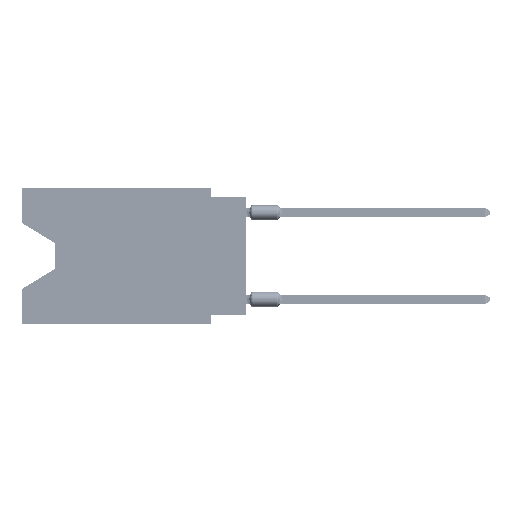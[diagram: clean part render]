
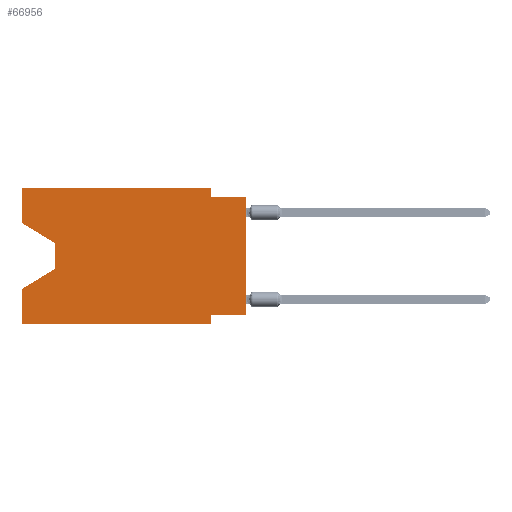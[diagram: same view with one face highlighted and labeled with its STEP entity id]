
A CAD part, left-side view. The second image highlights one B-rep face of the part: STEP entity #66956.
In plain terms, the highlighted planar face has unit normal (-1, 0, 0).
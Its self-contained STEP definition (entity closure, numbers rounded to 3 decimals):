
#85 = ORIENTED_EDGE ( 'NONE', *, *, #61911, .T. ) ;
#291 = CARTESIAN_POINT ( 'NONE',  ( 0., 2.54, 0. ) ) ;
#865 = LINE ( 'NONE', #1725, #47856 ) ;
#953 = ORIENTED_EDGE ( 'NONE', *, *, #16409, .F. ) ;
#1725 = CARTESIAN_POINT ( 'NONE',  ( 0., 2.54, -9.906 ) ) ;
#3393 = ORIENTED_EDGE ( 'NONE', *, *, #36086, .F. ) ;
#3420 = LINE ( 'NONE', #84178, #83410 ) ;
#5322 = CARTESIAN_POINT ( 'NONE',  ( 0., 13.97, -4.013 ) ) ;
#5913 = DIRECTION ( 'NONE',  ( 0., 0., -1. ) ) ;
#6177 = DIRECTION ( 'NONE',  ( 0., 0., -1. ) ) ;
#7702 = CARTESIAN_POINT ( 'NONE',  ( 0., 0., -0.635 ) ) ;
#8508 = DIRECTION ( 'NONE',  ( 0., -0.855, -0.519 ) ) ;
#9386 = CARTESIAN_POINT ( 'NONE',  ( 0., 0., 0. ) ) ;
#10433 = EDGE_CURVE ( 'NONE', #34516, #54500, #32031, .T. ) ;
#11161 = CARTESIAN_POINT ( 'NONE',  ( 0., 2.54, 0. ) ) ;
#11416 = LINE ( 'NONE', #5322, #69441 ) ;
#11665 = VECTOR ( 'NONE', #34186, 1000. ) ;
#12530 = VERTEX_POINT ( 'NONE', #73570 ) ;
#13395 = VECTOR ( 'NONE', #21501, 1000. ) ;
#13916 = DIRECTION ( 'NONE',  ( 0., 0., -1. ) ) ;
#15019 = CARTESIAN_POINT ( 'NONE',  ( 0., 16.383, -2.546 ) ) ;
#16210 = EDGE_CURVE ( 'NONE', #38763, #74793, #22685, .T. ) ;
#16409 = EDGE_CURVE ( 'NONE', #73768, #19472, #865, .T. ) ;
#19472 = VERTEX_POINT ( 'NONE', #46009 ) ;
#21501 = DIRECTION ( 'NONE',  ( 0., 0., 1. ) ) ;
#21680 = VECTOR ( 'NONE', #58626, 1000. ) ;
#22216 = ORIENTED_EDGE ( 'NONE', *, *, #10433, .F. ) ;
#22685 = LINE ( 'NONE', #36582, #36771 ) ;
#24603 = CARTESIAN_POINT ( 'NONE',  ( 0., 0., -0.635 ) ) ;
#25731 = VECTOR ( 'NONE', #8508, 1000. ) ;
#26202 = VERTEX_POINT ( 'NONE', #66694 ) ;
#26262 = EDGE_CURVE ( 'NONE', #26202, #38763, #81428, .T. ) ;
#26643 = CARTESIAN_POINT ( 'NONE',  ( 0., 16.383, -9.906 ) ) ;
#27681 = DIRECTION ( 'NONE',  ( 0., 0., -1. ) ) ;
#28984 = VERTEX_POINT ( 'NONE', #60404 ) ;
#29018 = VECTOR ( 'NONE', #39448, 1000. ) ;
#30464 = ORIENTED_EDGE ( 'NONE', *, *, #26262, .F. ) ;
#31731 = ORIENTED_EDGE ( 'NONE', *, *, #72070, .T. ) ;
#32031 = LINE ( 'NONE', #58087, #45026 ) ;
#32732 = EDGE_LOOP ( 'NONE', ( #79711, #31731, #55553, #22216, #79276, #953, #46967, #85, #33326, #3393, #66245, #30464 ) ) ;
#33326 = ORIENTED_EDGE ( 'NONE', *, *, #43011, .F. ) ;
#33374 = VERTEX_POINT ( 'NONE', #85211 ) ;
#34186 = DIRECTION ( 'NONE',  ( 0., -1., 0. ) ) ;
#34516 = VERTEX_POINT ( 'NONE', #26643 ) ;
#36086 = EDGE_CURVE ( 'NONE', #74793, #12530, #65415, .T. ) ;
#36582 = CARTESIAN_POINT ( 'NONE',  ( 0., 16.383, 0. ) ) ;
#36771 = VECTOR ( 'NONE', #69169, 1000. ) ;
#38481 = VERTEX_POINT ( 'NONE', #24603 ) ;
#38763 = VERTEX_POINT ( 'NONE', #68850 ) ;
#39448 = DIRECTION ( 'NONE',  ( 0., 0.855, -0.519 ) ) ;
#41419 = LINE ( 'NONE', #81353, #21680 ) ;
#41941 = LINE ( 'NONE', #9386, #58423 ) ;
#41967 = CARTESIAN_POINT ( 'NONE',  ( 0., 16.383, -7.36 ) ) ;
#43011 = EDGE_CURVE ( 'NONE', #12530, #38481, #74551, .T. ) ;
#45026 = VECTOR ( 'NONE', #58510, 1000. ) ;
#46009 = CARTESIAN_POINT ( 'NONE',  ( 0., 2.54, -9.906 ) ) ;
#46384 = CARTESIAN_POINT ( 'NONE',  ( 0., 16.383, 0. ) ) ;
#46967 = ORIENTED_EDGE ( 'NONE', *, *, #79186, .F. ) ;
#47856 = VECTOR ( 'NONE', #13916, 1000. ) ;
#48050 = LINE ( 'NONE', #15019, #25731 ) ;
#50352 = DIRECTION ( 'NONE',  ( 0., -1., 0. ) ) ;
#53119 = VERTEX_POINT ( 'NONE', #83797 ) ;
#54500 = VERTEX_POINT ( 'NONE', #41967 ) ;
#55553 = ORIENTED_EDGE ( 'NONE', *, *, #57346, .T. ) ;
#57346 = EDGE_CURVE ( 'NONE', #53119, #54500, #85060, .T. ) ;
#58087 = CARTESIAN_POINT ( 'NONE',  ( 0., 16.383, 0. ) ) ;
#58423 = VECTOR ( 'NONE', #81465, 1000. ) ;
#58510 = DIRECTION ( 'NONE',  ( 0., 0., 1. ) ) ;
#58626 = DIRECTION ( 'NONE',  ( 0., 1., 0. ) ) ;
#59483 = PLANE ( 'NONE',  #83927 ) ;
#60404 = CARTESIAN_POINT ( 'NONE',  ( 0., 0., -9.271 ) ) ;
#61766 = EDGE_CURVE ( 'NONE', #34516, #19472, #3420, .T. ) ;
#61911 = EDGE_CURVE ( 'NONE', #28984, #38481, #41941, .T. ) ;
#65415 = LINE ( 'NONE', #11161, #83431 ) ;
#66245 = ORIENTED_EDGE ( 'NONE', *, *, #16210, .F. ) ;
#66694 = CARTESIAN_POINT ( 'NONE',  ( 0., 16.383, -2.546 ) ) ;
#66956 = ADVANCED_FACE ( 'NONE', ( #73276 ), #59483, .F. ) ;
#68361 = CARTESIAN_POINT ( 'NONE',  ( 0., 2.54, -9.271 ) ) ;
#68850 = CARTESIAN_POINT ( 'NONE',  ( 0., 16.383, 0. ) ) ;
#69169 = DIRECTION ( 'NONE',  ( 0., -1., 0. ) ) ;
#69441 = VECTOR ( 'NONE', #6177, 1000. ) ;
#72070 = EDGE_CURVE ( 'NONE', #33374, #53119, #11416, .T. ) ;
#73276 = FACE_OUTER_BOUND ( 'NONE', #32732, .T. ) ;
#73570 = CARTESIAN_POINT ( 'NONE',  ( 0., 2.54, -0.635 ) ) ;
#73768 = VERTEX_POINT ( 'NONE', #68361 ) ;
#74471 = CARTESIAN_POINT ( 'NONE',  ( 0., 16.383, 0. ) ) ;
#74551 = LINE ( 'NONE', #7702, #11665 ) ;
#74793 = VERTEX_POINT ( 'NONE', #291 ) ;
#78519 = EDGE_CURVE ( 'NONE', #26202, #33374, #48050, .T. ) ;
#79186 = EDGE_CURVE ( 'NONE', #28984, #73768, #41419, .T. ) ;
#79276 = ORIENTED_EDGE ( 'NONE', *, *, #61766, .T. ) ;
#79711 = ORIENTED_EDGE ( 'NONE', *, *, #78519, .T. ) ;
#79796 = CARTESIAN_POINT ( 'NONE',  ( 0., 13.97, -5.893 ) ) ;
#80641 = DIRECTION ( 'NONE',  ( 1., 0., 0. ) ) ;
#81353 = CARTESIAN_POINT ( 'NONE',  ( 0., 0., -9.271 ) ) ;
#81428 = LINE ( 'NONE', #74471, #13395 ) ;
#81465 = DIRECTION ( 'NONE',  ( 0., 0., 1. ) ) ;
#83410 = VECTOR ( 'NONE', #50352, 1000. ) ;
#83431 = VECTOR ( 'NONE', #5913, 1000. ) ;
#83797 = CARTESIAN_POINT ( 'NONE',  ( 0., 13.97, -5.893 ) ) ;
#83927 = AXIS2_PLACEMENT_3D ( 'NONE', #46384, #80641, #27681 ) ;
#84178 = CARTESIAN_POINT ( 'NONE',  ( 0., 16.383, -9.906 ) ) ;
#85060 = LINE ( 'NONE', #79796, #29018 ) ;
#85211 = CARTESIAN_POINT ( 'NONE',  ( 0., 13.97, -4.013 ) ) ;
